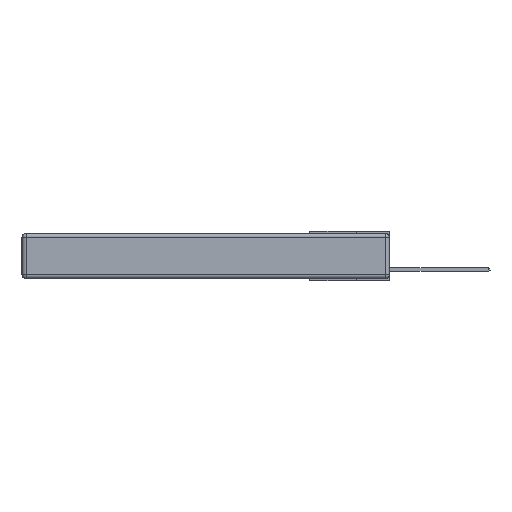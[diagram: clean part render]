
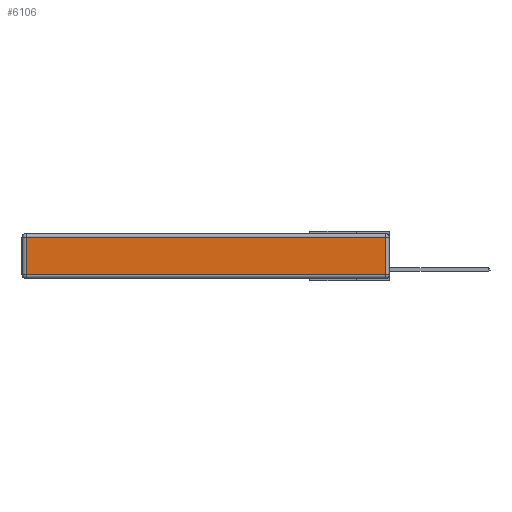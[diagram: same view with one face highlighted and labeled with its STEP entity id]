
A CAD part, left-side view. The second image highlights one B-rep face of the part: STEP entity #6106.
In plain terms, the highlighted planar face has unit normal (-1, 0, 0).
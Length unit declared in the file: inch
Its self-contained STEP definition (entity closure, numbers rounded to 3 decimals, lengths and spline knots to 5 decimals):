
#373 = DIRECTION ( 'NONE',  ( 0., -1., 0. ) ) ;
#1432 = FACE_OUTER_BOUND ( 'NONE', #14480, .T. ) ;
#1471 = EDGE_CURVE ( 'NONE', #1615, #16970, #4886, .T. ) ;
#1615 = VERTEX_POINT ( 'NONE', #9868 ) ;
#2455 = DIRECTION ( 'NONE',  ( 0., 0., 1. ) ) ;
#2996 = CARTESIAN_POINT ( 'NONE',  ( 0., 2.75, -0.03 ) ) ;
#3197 = CARTESIAN_POINT ( 'NONE',  ( 0., 0.03, -0.313 ) ) ;
#4368 = ORIENTED_EDGE ( 'NONE', *, *, #4606, .T. ) ;
#4606 = EDGE_CURVE ( 'NONE', #16970, #17922, #18267, .T. ) ;
#4741 = CARTESIAN_POINT ( 'NONE',  ( 0., 0., -0.313 ) ) ;
#4886 = LINE ( 'NONE', #4741, #6993 ) ;
#5603 = CARTESIAN_POINT ( 'NONE',  ( 0., 0.03, -0.343 ) ) ;
#5841 = PLANE ( 'NONE',  #19035 ) ;
#5907 = LINE ( 'NONE', #9358, #7073 ) ;
#6106 = ADVANCED_FACE ( 'NONE', ( #1432 ), #5841, .T. ) ;
#6479 = ORIENTED_EDGE ( 'NONE', *, *, #10354, .T. ) ;
#6708 = ORIENTED_EDGE ( 'NONE', *, *, #1471, .T. ) ;
#6993 = VECTOR ( 'NONE', #373, 39.37008 ) ;
#7073 = VECTOR ( 'NONE', #16826, 39.37008 ) ;
#7736 = ORIENTED_EDGE ( 'NONE', *, *, #18358, .T. ) ;
#7844 = VERTEX_POINT ( 'NONE', #9264 ) ;
#9264 = CARTESIAN_POINT ( 'NONE',  ( 0., 2.72, -0.03 ) ) ;
#9358 = CARTESIAN_POINT ( 'NONE',  ( 0., 2.72, -0.343 ) ) ;
#9868 = CARTESIAN_POINT ( 'NONE',  ( 0., 2.72, -0.313 ) ) ;
#10354 = EDGE_CURVE ( 'NONE', #7844, #1615, #5907, .T. ) ;
#10827 = VECTOR ( 'NONE', #2455, 39.37008 ) ;
#13431 = DIRECTION ( 'NONE',  ( 0., 1., 0. ) ) ;
#14480 = EDGE_LOOP ( 'NONE', ( #6708, #4368, #7736, #6479 ) ) ;
#14807 = DIRECTION ( 'NONE',  ( -1., 0., 0. ) ) ;
#15123 = CARTESIAN_POINT ( 'NONE',  ( 0., 0.03, -0.03 ) ) ;
#16243 = CARTESIAN_POINT ( 'NONE',  ( 0., 0., -0.343 ) ) ;
#16826 = DIRECTION ( 'NONE',  ( 0., 0., -1. ) ) ;
#16970 = VERTEX_POINT ( 'NONE', #3197 ) ;
#17815 = DIRECTION ( 'NONE',  ( 0., 0., 1. ) ) ;
#17922 = VERTEX_POINT ( 'NONE', #15123 ) ;
#18267 = LINE ( 'NONE', #5603, #10827 ) ;
#18358 = EDGE_CURVE ( 'NONE', #17922, #7844, #18450, .T. ) ;
#18450 = LINE ( 'NONE', #2996, #19168 ) ;
#19035 = AXIS2_PLACEMENT_3D ( 'NONE', #16243, #14807, #17815 ) ;
#19168 = VECTOR ( 'NONE', #13431, 39.37008 ) ;
